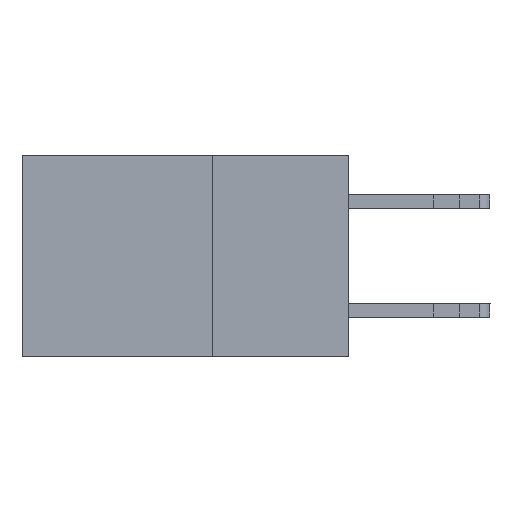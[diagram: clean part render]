
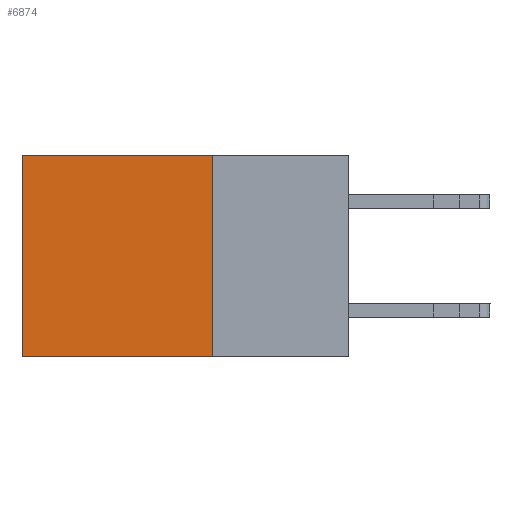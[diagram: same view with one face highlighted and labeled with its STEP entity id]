
A CAD part, left-side view. The second image highlights one B-rep face of the part: STEP entity #6874.
In plain terms, the highlighted planar face has unit normal (-1, 0, 0).
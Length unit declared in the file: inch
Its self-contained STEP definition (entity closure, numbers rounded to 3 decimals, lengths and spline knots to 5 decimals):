
#197 = EDGE_LOOP ( 'NONE', ( #5447, #9030, #8817, #9252 ) ) ;
#309 = VERTEX_POINT ( 'NONE', #3468 ) ;
#455 = FACE_OUTER_BOUND ( 'NONE', #197, .T. ) ;
#1225 = CARTESIAN_POINT ( 'NONE',  ( 0.2615, 0.6, -0.37 ) ) ;
#1301 = EDGE_CURVE ( 'NONE', #5438, #7046, #8183, .T. ) ;
#1365 = VERTEX_POINT ( 'NONE', #7813 ) ;
#2829 = VECTOR ( 'NONE', #7464, 39.37008 ) ;
#2981 = LINE ( 'NONE', #8416, #6960 ) ;
#3309 = EDGE_CURVE ( 'NONE', #7046, #1365, #3676, .T. ) ;
#3468 = CARTESIAN_POINT ( 'NONE',  ( 0.2615, 0.6, 0. ) ) ;
#3676 = LINE ( 'NONE', #9395, #5611 ) ;
#3903 = AXIS2_PLACEMENT_3D ( 'NONE', #5674, #9539, #4849 ) ;
#4062 = PLANE ( 'NONE',  #3903 ) ;
#4849 = DIRECTION ( 'NONE',  ( 0., 0., -1. ) ) ;
#5438 = VERTEX_POINT ( 'NONE', #9594 ) ;
#5447 = ORIENTED_EDGE ( 'NONE', *, *, #5545, .T. ) ;
#5545 = EDGE_CURVE ( 'NONE', #309, #1365, #7552, .T. ) ;
#5611 = VECTOR ( 'NONE', #10156, 39.37008 ) ;
#5674 = CARTESIAN_POINT ( 'NONE',  ( 0.2615, 0.25, -0.37 ) ) ;
#6345 = EDGE_CURVE ( 'NONE', #5438, #309, #2981, .T. ) ;
#6874 = ADVANCED_FACE ( 'NONE', ( #455 ), #4062, .F. ) ;
#6960 = VECTOR ( 'NONE', #9130, 39.37008 ) ;
#7046 = VERTEX_POINT ( 'NONE', #10430 ) ;
#7464 = DIRECTION ( 'NONE',  ( 0., 0., -1. ) ) ;
#7552 = LINE ( 'NONE', #1225, #2829 ) ;
#7813 = CARTESIAN_POINT ( 'NONE',  ( 0.2615, 0.6, -0.37 ) ) ;
#8183 = LINE ( 'NONE', #10927, #10161 ) ;
#8370 = DIRECTION ( 'NONE',  ( 0., 0., -1. ) ) ;
#8416 = CARTESIAN_POINT ( 'NONE',  ( 0.2615, 0.25, 0. ) ) ;
#8817 = ORIENTED_EDGE ( 'NONE', *, *, #1301, .F. ) ;
#9030 = ORIENTED_EDGE ( 'NONE', *, *, #3309, .F. ) ;
#9130 = DIRECTION ( 'NONE',  ( 0., 1., 0. ) ) ;
#9252 = ORIENTED_EDGE ( 'NONE', *, *, #6345, .T. ) ;
#9395 = CARTESIAN_POINT ( 'NONE',  ( 0.2615, 0.25, -0.37 ) ) ;
#9539 = DIRECTION ( 'NONE',  ( 1., 0., 0. ) ) ;
#9594 = CARTESIAN_POINT ( 'NONE',  ( 0.2615, 0.25, 0. ) ) ;
#10156 = DIRECTION ( 'NONE',  ( 0., 1., 0. ) ) ;
#10161 = VECTOR ( 'NONE', #8370, 39.37008 ) ;
#10430 = CARTESIAN_POINT ( 'NONE',  ( 0.2615, 0.25, -0.37 ) ) ;
#10927 = CARTESIAN_POINT ( 'NONE',  ( 0.2615, 0.25, -0.37 ) ) ;
